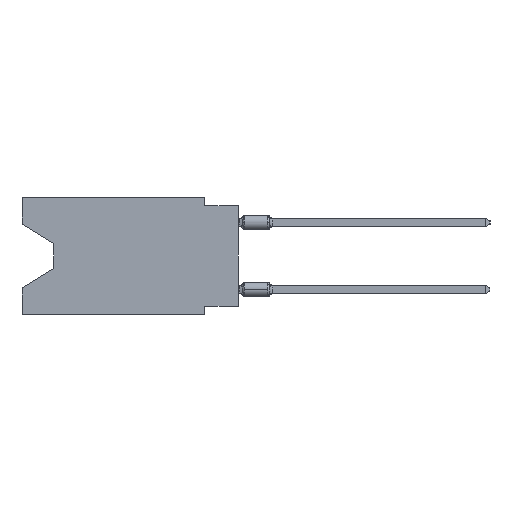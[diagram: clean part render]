
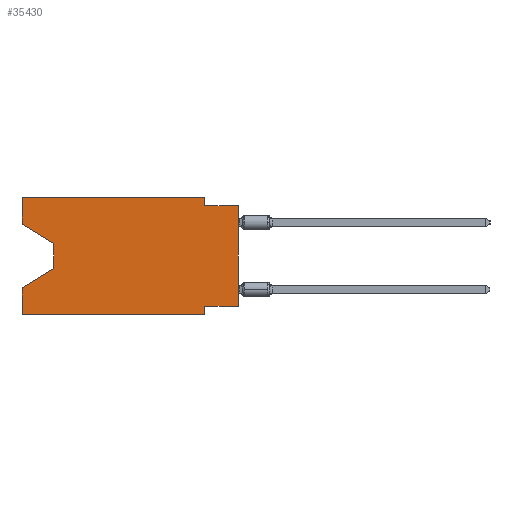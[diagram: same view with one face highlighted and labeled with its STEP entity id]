
A CAD part, left-side view. The second image highlights one B-rep face of the part: STEP entity #35430.
In plain terms, the highlighted planar face has unit normal (-1, 0, 0).
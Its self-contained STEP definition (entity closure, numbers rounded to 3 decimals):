
#36 = VECTOR ( 'NONE', #17610, 1000. ) ;
#137 = CARTESIAN_POINT ( 'NONE',  ( 0., 2.54, 0. ) ) ;
#265 = VECTOR ( 'NONE', #1899, 1000. ) ;
#346 = VECTOR ( 'NONE', #38129, 1000. ) ;
#1057 = AXIS2_PLACEMENT_3D ( 'NONE', #27805, #1318, #13690 ) ;
#1318 = DIRECTION ( 'NONE',  ( 1., 0., 0. ) ) ;
#1411 = CARTESIAN_POINT ( 'NONE',  ( 0., 16.383, -2.038 ) ) ;
#1491 = VECTOR ( 'NONE', #29541, 1000. ) ;
#1580 = CARTESIAN_POINT ( 'NONE',  ( 0., 16.383, -6.852 ) ) ;
#1762 = ORIENTED_EDGE ( 'NONE', *, *, #24047, .T. ) ;
#1899 = DIRECTION ( 'NONE',  ( 0., 0.855, -0.519 ) ) ;
#2311 = VERTEX_POINT ( 'NONE', #3452 ) ;
#2614 = EDGE_LOOP ( 'NONE', ( #38073, #2741, #1762, #6071, #7772, #28279, #22386, #5041, #31914, #3844, #23430, #13126 ) ) ;
#2645 = EDGE_CURVE ( 'NONE', #23632, #23657, #5917, .T. ) ;
#2646 = LINE ( 'NONE', #34942, #4404 ) ;
#2649 = EDGE_CURVE ( 'NONE', #10193, #22936, #26653, .T. ) ;
#2716 = LINE ( 'NONE', #14509, #346 ) ;
#2741 = ORIENTED_EDGE ( 'NONE', *, *, #5231, .T. ) ;
#3452 = CARTESIAN_POINT ( 'NONE',  ( 0., 16.383, -8.89 ) ) ;
#3680 = CARTESIAN_POINT ( 'NONE',  ( 0., 16.383, 0. ) ) ;
#3844 = ORIENTED_EDGE ( 'NONE', *, *, #2649, .F. ) ;
#4404 = VECTOR ( 'NONE', #23547, 1000. ) ;
#4425 = CARTESIAN_POINT ( 'NONE',  ( 0., 16.383, 0. ) ) ;
#5041 = ORIENTED_EDGE ( 'NONE', *, *, #18804, .T. ) ;
#5091 = EDGE_CURVE ( 'NONE', #28543, #23632, #2646, .T. ) ;
#5231 = EDGE_CURVE ( 'NONE', #8443, #9051, #35718, .T. ) ;
#5391 = VECTOR ( 'NONE', #26209, 1000. ) ;
#5917 = LINE ( 'NONE', #32623, #1491 ) ;
#5994 = DIRECTION ( 'NONE',  ( 0., 0., 1. ) ) ;
#6071 = ORIENTED_EDGE ( 'NONE', *, *, #31305, .F. ) ;
#7284 = CARTESIAN_POINT ( 'NONE',  ( 0., 16.383, -8.89 ) ) ;
#7577 = CARTESIAN_POINT ( 'NONE',  ( 0., 2.54, -8.255 ) ) ;
#7772 = ORIENTED_EDGE ( 'NONE', *, *, #28407, .T. ) ;
#8443 = VERTEX_POINT ( 'NONE', #36709 ) ;
#9051 = VERTEX_POINT ( 'NONE', #34137 ) ;
#9384 = DIRECTION ( 'NONE',  ( 0., 0., -1. ) ) ;
#9502 = VERTEX_POINT ( 'NONE', #12350 ) ;
#9561 = CARTESIAN_POINT ( 'NONE',  ( 0., 13.97, -3.505 ) ) ;
#10193 = VERTEX_POINT ( 'NONE', #16342 ) ;
#10584 = EDGE_CURVE ( 'NONE', #9502, #8443, #33519, .T. ) ;
#12350 = CARTESIAN_POINT ( 'NONE',  ( 0., 16.383, -2.038 ) ) ;
#13126 = ORIENTED_EDGE ( 'NONE', *, *, #33902, .F. ) ;
#13151 = CARTESIAN_POINT ( 'NONE',  ( 0., 16.383, 0. ) ) ;
#13690 = DIRECTION ( 'NONE',  ( 0., 0., -1. ) ) ;
#14405 = LINE ( 'NONE', #35114, #5391 ) ;
#14509 = CARTESIAN_POINT ( 'NONE',  ( 0., 0., 0. ) ) ;
#15082 = CARTESIAN_POINT ( 'NONE',  ( 0., 16.383, 0. ) ) ;
#15424 = DIRECTION ( 'NONE',  ( 0., 0., -1. ) ) ;
#15631 = LINE ( 'NONE', #7284, #33858 ) ;
#16017 = FACE_OUTER_BOUND ( 'NONE', #2614, .T. ) ;
#16060 = LINE ( 'NONE', #13151, #20760 ) ;
#16342 = CARTESIAN_POINT ( 'NONE',  ( 0., 2.54, 0. ) ) ;
#17610 = DIRECTION ( 'NONE',  ( 0., 0., 1. ) ) ;
#18804 = EDGE_CURVE ( 'NONE', #28543, #28616, #2716, .T. ) ;
#19440 = EDGE_CURVE ( 'NONE', #37659, #10193, #16060, .T. ) ;
#20760 = VECTOR ( 'NONE', #36172, 1000. ) ;
#22015 = LINE ( 'NONE', #37120, #265 ) ;
#22386 = ORIENTED_EDGE ( 'NONE', *, *, #5091, .F. ) ;
#22936 = VERTEX_POINT ( 'NONE', #26627 ) ;
#23340 = CARTESIAN_POINT ( 'NONE',  ( 0., 0., -0.635 ) ) ;
#23430 = ORIENTED_EDGE ( 'NONE', *, *, #19440, .F. ) ;
#23547 = DIRECTION ( 'NONE',  ( 0., 1., 0. ) ) ;
#23632 = VERTEX_POINT ( 'NONE', #7577 ) ;
#23657 = VERTEX_POINT ( 'NONE', #23775 ) ;
#23775 = CARTESIAN_POINT ( 'NONE',  ( 0., 2.54, -8.89 ) ) ;
#23800 = LINE ( 'NONE', #3680, #35552 ) ;
#24047 = EDGE_CURVE ( 'NONE', #9051, #30492, #22015, .T. ) ;
#25826 = EDGE_CURVE ( 'NONE', #22936, #28616, #14405, .T. ) ;
#26204 = VECTOR ( 'NONE', #15424, 1000. ) ;
#26209 = DIRECTION ( 'NONE',  ( 0., -1., 0. ) ) ;
#26627 = CARTESIAN_POINT ( 'NONE',  ( 0., 2.54, -0.635 ) ) ;
#26653 = LINE ( 'NONE', #137, #26204 ) ;
#27147 = DIRECTION ( 'NONE',  ( 0., -0.855, -0.519 ) ) ;
#27805 = CARTESIAN_POINT ( 'NONE',  ( 0., 16.383, 0. ) ) ;
#28279 = ORIENTED_EDGE ( 'NONE', *, *, #2645, .F. ) ;
#28407 = EDGE_CURVE ( 'NONE', #2311, #23657, #15631, .T. ) ;
#28543 = VERTEX_POINT ( 'NONE', #29886 ) ;
#28616 = VERTEX_POINT ( 'NONE', #23340 ) ;
#29541 = DIRECTION ( 'NONE',  ( 0., 0., -1. ) ) ;
#29886 = CARTESIAN_POINT ( 'NONE',  ( 0., 0., -8.255 ) ) ;
#30492 = VERTEX_POINT ( 'NONE', #1580 ) ;
#30502 = PLANE ( 'NONE',  #1057 ) ;
#30687 = DIRECTION ( 'NONE',  ( 0., -1., 0. ) ) ;
#31305 = EDGE_CURVE ( 'NONE', #2311, #30492, #32878, .T. ) ;
#31382 = VECTOR ( 'NONE', #27147, 1000. ) ;
#31914 = ORIENTED_EDGE ( 'NONE', *, *, #25826, .F. ) ;
#32170 = VECTOR ( 'NONE', #9384, 1000. ) ;
#32623 = CARTESIAN_POINT ( 'NONE',  ( 0., 2.54, -8.89 ) ) ;
#32878 = LINE ( 'NONE', #15082, #36 ) ;
#33519 = LINE ( 'NONE', #1411, #31382 ) ;
#33858 = VECTOR ( 'NONE', #30687, 1000. ) ;
#33902 = EDGE_CURVE ( 'NONE', #9502, #37659, #23800, .T. ) ;
#34137 = CARTESIAN_POINT ( 'NONE',  ( 0., 13.97, -5.385 ) ) ;
#34942 = CARTESIAN_POINT ( 'NONE',  ( 0., 0., -8.255 ) ) ;
#35114 = CARTESIAN_POINT ( 'NONE',  ( 0., 0., -0.635 ) ) ;
#35430 = ADVANCED_FACE ( 'NONE', ( #16017 ), #30502, .F. ) ;
#35552 = VECTOR ( 'NONE', #5994, 1000. ) ;
#35718 = LINE ( 'NONE', #9561, #32170 ) ;
#36172 = DIRECTION ( 'NONE',  ( 0., -1., 0. ) ) ;
#36709 = CARTESIAN_POINT ( 'NONE',  ( 0., 13.97, -3.505 ) ) ;
#37120 = CARTESIAN_POINT ( 'NONE',  ( 0., 13.97, -5.385 ) ) ;
#37659 = VERTEX_POINT ( 'NONE', #4425 ) ;
#38073 = ORIENTED_EDGE ( 'NONE', *, *, #10584, .T. ) ;
#38129 = DIRECTION ( 'NONE',  ( 0., 0., 1. ) ) ;
